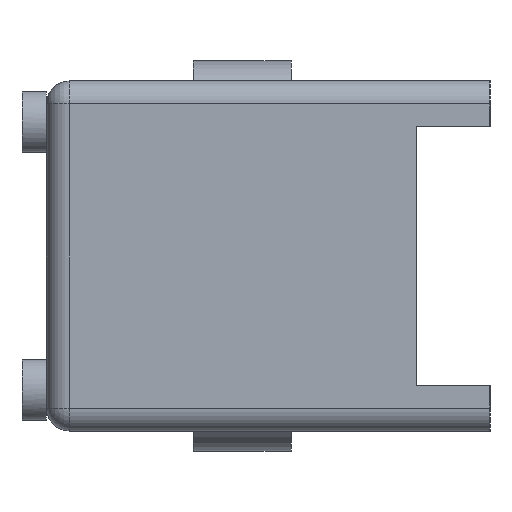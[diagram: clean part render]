
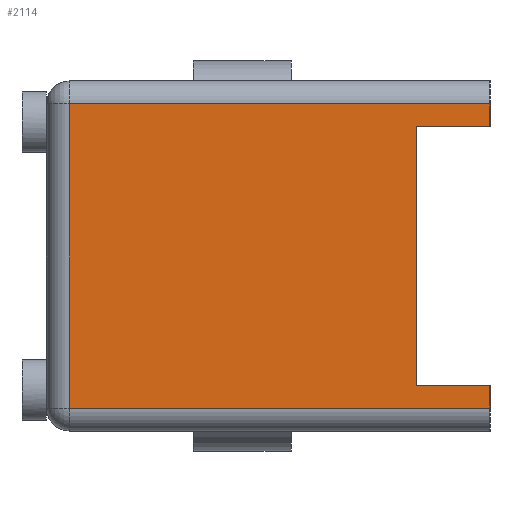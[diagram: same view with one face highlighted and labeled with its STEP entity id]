
A CAD part, left-side view. The second image highlights one B-rep face of the part: STEP entity #2114.
In plain terms, the highlighted planar face has unit normal (-1, 0, 0).
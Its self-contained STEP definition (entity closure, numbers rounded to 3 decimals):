
#3 = LINE ( 'NONE', #1083, #1896 ) ;
#21 = EDGE_CURVE ( 'NONE', #1313, #1923, #990, .T. ) ;
#24 = CARTESIAN_POINT ( 'NONE',  ( 0., 0., -18.161 ) ) ;
#53 = DIRECTION ( 'NONE',  ( 0., 1., 0. ) ) ;
#84 = CARTESIAN_POINT ( 'NONE',  ( 0., 0., -18.161 ) ) ;
#90 = CARTESIAN_POINT ( 'NONE',  ( 0., 3.81, -15.824 ) ) ;
#179 = CARTESIAN_POINT ( 'NONE',  ( 0., 0., -18.161 ) ) ;
#190 = PLANE ( 'NONE',  #1117 ) ;
#227 = VERTEX_POINT ( 'NONE', #1084 ) ;
#242 = DIRECTION ( 'NONE',  ( 0., -1., 0. ) ) ;
#262 = ORIENTED_EDGE ( 'NONE', *, *, #1520, .T. ) ;
#296 = EDGE_CURVE ( 'NONE', #1675, #2185, #1607, .T. ) ;
#298 = ORIENTED_EDGE ( 'NONE', *, *, #296, .T. ) ;
#356 = DIRECTION ( 'NONE',  ( 0., 0., 1. ) ) ;
#406 = CARTESIAN_POINT ( 'NONE',  ( 0., 0., -16.967 ) ) ;
#571 = VERTEX_POINT ( 'NONE', #1563 ) ;
#651 = ORIENTED_EDGE ( 'NONE', *, *, #21, .F. ) ;
#660 = DIRECTION ( 'NONE',  ( 0., 0., -1. ) ) ;
#671 = CARTESIAN_POINT ( 'NONE',  ( 0., 0., -1.194 ) ) ;
#688 = VERTEX_POINT ( 'NONE', #1478 ) ;
#757 = DIRECTION ( 'NONE',  ( 0., 0., 1. ) ) ;
#761 = DIRECTION ( 'NONE',  ( 0., -1., 0. ) ) ;
#791 = VECTOR ( 'NONE', #1639, 1000. ) ;
#885 = LINE ( 'NONE', #84, #1741 ) ;
#887 = EDGE_CURVE ( 'NONE', #571, #1675, #1992, .T. ) ;
#899 = ORIENTED_EDGE ( 'NONE', *, *, #887, .T. ) ;
#941 = CARTESIAN_POINT ( 'NONE',  ( 0., 21.819, -18.161 ) ) ;
#990 = LINE ( 'NONE', #2229, #2106 ) ;
#1018 = CARTESIAN_POINT ( 'NONE',  ( 0., 23.012, -1.194 ) ) ;
#1072 = ORIENTED_EDGE ( 'NONE', *, *, #2239, .F. ) ;
#1083 = CARTESIAN_POINT ( 'NONE',  ( 0., 3.81, -2.337 ) ) ;
#1084 = CARTESIAN_POINT ( 'NONE',  ( 0., 0., -15.824 ) ) ;
#1117 = AXIS2_PLACEMENT_3D ( 'NONE', #24, #1219, #1396 ) ;
#1219 = DIRECTION ( 'NONE',  ( -1., 0., 0. ) ) ;
#1254 = ORIENTED_EDGE ( 'NONE', *, *, #1591, .T. ) ;
#1313 = VERTEX_POINT ( 'NONE', #2064 ) ;
#1316 = VECTOR ( 'NONE', #1873, 1000. ) ;
#1335 = ORIENTED_EDGE ( 'NONE', *, *, #2001, .T. ) ;
#1364 = CARTESIAN_POINT ( 'NONE',  ( 0., 3.81, -15.824 ) ) ;
#1376 = CARTESIAN_POINT ( 'NONE',  ( 0., 21.819, -16.967 ) ) ;
#1396 = DIRECTION ( 'NONE',  ( 0., 0., 1. ) ) ;
#1404 = VECTOR ( 'NONE', #761, 1000. ) ;
#1434 = LINE ( 'NONE', #90, #1404 ) ;
#1478 = CARTESIAN_POINT ( 'NONE',  ( 0., 0., -2.337 ) ) ;
#1505 = EDGE_LOOP ( 'NONE', ( #899, #298, #1335, #1072, #651, #1532, #262, #1254 ) ) ;
#1520 = EDGE_CURVE ( 'NONE', #688, #2097, #885, .T. ) ;
#1532 = ORIENTED_EDGE ( 'NONE', *, *, #1628, .F. ) ;
#1563 = CARTESIAN_POINT ( 'NONE',  ( 0., 21.819, -1.194 ) ) ;
#1591 = EDGE_CURVE ( 'NONE', #2097, #571, #1689, .T. ) ;
#1607 = LINE ( 'NONE', #1788, #1908 ) ;
#1628 = EDGE_CURVE ( 'NONE', #688, #1313, #3, .T. ) ;
#1639 = DIRECTION ( 'NONE',  ( 0., 0., -1. ) ) ;
#1675 = VERTEX_POINT ( 'NONE', #1376 ) ;
#1689 = LINE ( 'NONE', #1018, #1316 ) ;
#1734 = FACE_OUTER_BOUND ( 'NONE', #1505, .T. ) ;
#1741 = VECTOR ( 'NONE', #757, 1000. ) ;
#1788 = CARTESIAN_POINT ( 'NONE',  ( 0., 0., -16.967 ) ) ;
#1873 = DIRECTION ( 'NONE',  ( 0., 1., 0. ) ) ;
#1888 = LINE ( 'NONE', #179, #2209 ) ;
#1896 = VECTOR ( 'NONE', #53, 1000. ) ;
#1908 = VECTOR ( 'NONE', #242, 1000. ) ;
#1923 = VERTEX_POINT ( 'NONE', #1364 ) ;
#1992 = LINE ( 'NONE', #941, #791 ) ;
#2001 = EDGE_CURVE ( 'NONE', #2185, #227, #1888, .T. ) ;
#2064 = CARTESIAN_POINT ( 'NONE',  ( 0., 3.81, -2.337 ) ) ;
#2097 = VERTEX_POINT ( 'NONE', #671 ) ;
#2106 = VECTOR ( 'NONE', #660, 1000. ) ;
#2114 = ADVANCED_FACE ( 'NONE', ( #1734 ), #190, .T. ) ;
#2185 = VERTEX_POINT ( 'NONE', #406 ) ;
#2209 = VECTOR ( 'NONE', #356, 1000. ) ;
#2229 = CARTESIAN_POINT ( 'NONE',  ( 0., 3.81, -15.824 ) ) ;
#2239 = EDGE_CURVE ( 'NONE', #1923, #227, #1434, .T. ) ;
